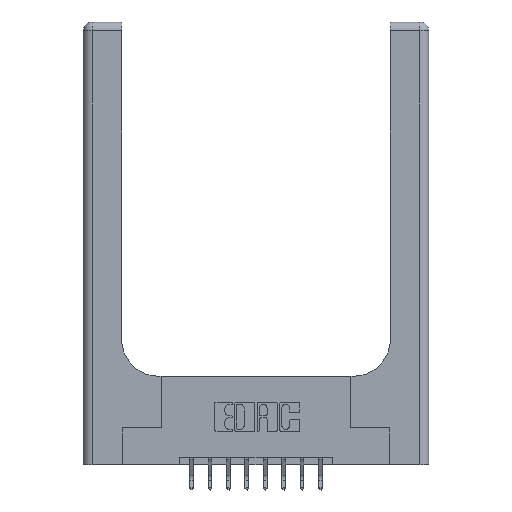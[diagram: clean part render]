
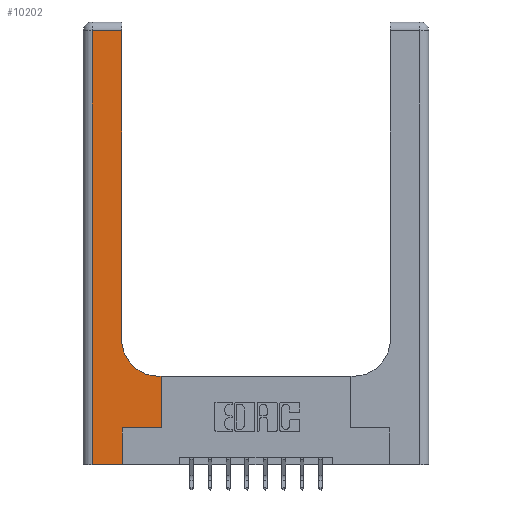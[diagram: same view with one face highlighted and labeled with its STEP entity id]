
A CAD part, top view. The second image highlights one B-rep face of the part: STEP entity #10202.
In plain terms, the highlighted planar face has unit normal (0, 0, 1).
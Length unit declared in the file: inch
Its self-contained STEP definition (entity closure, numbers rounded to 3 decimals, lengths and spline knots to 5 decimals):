
#303 = LINE ( 'NONE', #11230, #5489 ) ;
#729 = VECTOR ( 'NONE', #3623, 39.37008 ) ;
#952 = EDGE_CURVE ( 'NONE', #15078, #9808, #13751, .T. ) ;
#1310 = ORIENTED_EDGE ( 'NONE', *, *, #13194, .T. ) ;
#1444 = DIRECTION ( 'NONE',  ( 0., 1., 0. ) ) ;
#1522 = CARTESIAN_POINT ( 'NONE',  ( 0., 0., 0.37 ) ) ;
#1782 = CARTESIAN_POINT ( 'NONE',  ( 0.265, 0., 0.37 ) ) ;
#1829 = EDGE_CURVE ( 'NONE', #14123, #10329, #3282, .T. ) ;
#2497 = ORIENTED_EDGE ( 'NONE', *, *, #7614, .T. ) ;
#2545 = CARTESIAN_POINT ( 'NONE',  ( 0.265, 0.25, 0.37 ) ) ;
#2578 = EDGE_LOOP ( 'NONE', ( #7076, #1310, #2497, #11258, #5785, #10426, #13328, #14172, #7221 ) ) ;
#2720 = DIRECTION ( 'NONE',  ( 0., 1., 0. ) ) ;
#3282 = LINE ( 'NONE', #4971, #3464 ) ;
#3456 = CARTESIAN_POINT ( 'NONE',  ( 0.51, 0.6, 0.37 ) ) ;
#3464 = VECTOR ( 'NONE', #1444, 39.37008 ) ;
#3581 = VERTEX_POINT ( 'NONE', #14454 ) ;
#3623 = DIRECTION ( 'NONE',  ( 1., 0., 0. ) ) ;
#3848 = CIRCLE ( 'NONE', #10645, 0.25 ) ;
#4052 = CARTESIAN_POINT ( 'NONE',  ( 0.26, 0.6, 0.37 ) ) ;
#4129 = DIRECTION ( 'NONE',  ( 0., 1., 0. ) ) ;
#4152 = DIRECTION ( 'NONE',  ( -1., 0., 0. ) ) ;
#4184 = CARTESIAN_POINT ( 'NONE',  ( 0., 3., 0.37 ) ) ;
#4971 = CARTESIAN_POINT ( 'NONE',  ( 0.26, 3., 0.37 ) ) ;
#5489 = VECTOR ( 'NONE', #4129, 39.37008 ) ;
#5581 = CARTESIAN_POINT ( 'NONE',  ( 0.26, 2.94, 0.37 ) ) ;
#5785 = ORIENTED_EDGE ( 'NONE', *, *, #6440, .T. ) ;
#6237 = CARTESIAN_POINT ( 'NONE',  ( 0.528, 0.25, 0.37 ) ) ;
#6440 = EDGE_CURVE ( 'NONE', #6472, #15078, #303, .T. ) ;
#6472 = VERTEX_POINT ( 'NONE', #1782 ) ;
#6755 = AXIS2_PLACEMENT_3D ( 'NONE', #4184, #12388, #8921 ) ;
#6805 = CARTESIAN_POINT ( 'NONE',  ( 0.528, 0.6, 0.37 ) ) ;
#7043 = DIRECTION ( 'NONE',  ( 1., 0., 0. ) ) ;
#7076 = ORIENTED_EDGE ( 'NONE', *, *, #1829, .T. ) ;
#7221 = ORIENTED_EDGE ( 'NONE', *, *, #10772, .T. ) ;
#7222 = VECTOR ( 'NONE', #4152, 39.37008 ) ;
#7394 = FACE_OUTER_BOUND ( 'NONE', #2578, .T. ) ;
#7455 = DIRECTION ( 'NONE',  ( -1., 0., 0. ) ) ;
#7469 = DIRECTION ( 'NONE',  ( 0., -1., 0. ) ) ;
#7614 = EDGE_CURVE ( 'NONE', #3581, #13127, #10199, .T. ) ;
#7657 = DIRECTION ( 'NONE',  ( 1., 0., 0. ) ) ;
#8317 = LINE ( 'NONE', #4052, #7222 ) ;
#8325 = CARTESIAN_POINT ( 'NONE',  ( 0.528, 0.25, 0.37 ) ) ;
#8884 = CARTESIAN_POINT ( 'NONE',  ( 0.26, 0.85, 0.37 ) ) ;
#8921 = DIRECTION ( 'NONE',  ( -1., 0., 0. ) ) ;
#9393 = EDGE_CURVE ( 'NONE', #11562, #14294, #8317, .T. ) ;
#9660 = CARTESIAN_POINT ( 'NONE',  ( 0.06, 3., 0.37 ) ) ;
#9759 = CARTESIAN_POINT ( 'NONE',  ( 0., 2.94, 0.37 ) ) ;
#9808 = VERTEX_POINT ( 'NONE', #8325 ) ;
#10199 = LINE ( 'NONE', #9660, #11870 ) ;
#10202 = ADVANCED_FACE ( 'NONE', ( #7394 ), #11188, .F. ) ;
#10329 = VERTEX_POINT ( 'NONE', #5581 ) ;
#10426 = ORIENTED_EDGE ( 'NONE', *, *, #952, .T. ) ;
#10645 = AXIS2_PLACEMENT_3D ( 'NONE', #12807, #12859, #7043 ) ;
#10772 = EDGE_CURVE ( 'NONE', #14294, #14123, #3848, .T. ) ;
#11188 = PLANE ( 'NONE',  #6755 ) ;
#11230 = CARTESIAN_POINT ( 'NONE',  ( 0.265, 0., 0.37 ) ) ;
#11258 = ORIENTED_EDGE ( 'NONE', *, *, #14582, .T. ) ;
#11562 = VERTEX_POINT ( 'NONE', #6805 ) ;
#11677 = CARTESIAN_POINT ( 'NONE',  ( 0.265, 0.25, 0.37 ) ) ;
#11870 = VECTOR ( 'NONE', #7469, 39.37008 ) ;
#12375 = VECTOR ( 'NONE', #7657, 39.37008 ) ;
#12388 = DIRECTION ( 'NONE',  ( 0., 0., -1. ) ) ;
#12807 = CARTESIAN_POINT ( 'NONE',  ( 0.51, 0.85, 0.37 ) ) ;
#12859 = DIRECTION ( 'NONE',  ( 0., 0., -1. ) ) ;
#13098 = LINE ( 'NONE', #6237, #13461 ) ;
#13127 = VERTEX_POINT ( 'NONE', #14638 ) ;
#13194 = EDGE_CURVE ( 'NONE', #10329, #3581, #13651, .T. ) ;
#13328 = ORIENTED_EDGE ( 'NONE', *, *, #13518, .T. ) ;
#13461 = VECTOR ( 'NONE', #2720, 39.37008 ) ;
#13518 = EDGE_CURVE ( 'NONE', #9808, #11562, #13098, .T. ) ;
#13651 = LINE ( 'NONE', #9759, #14223 ) ;
#13751 = LINE ( 'NONE', #11677, #729 ) ;
#14123 = VERTEX_POINT ( 'NONE', #8884 ) ;
#14172 = ORIENTED_EDGE ( 'NONE', *, *, #9393, .T. ) ;
#14223 = VECTOR ( 'NONE', #7455, 39.37008 ) ;
#14294 = VERTEX_POINT ( 'NONE', #3456 ) ;
#14387 = LINE ( 'NONE', #1522, #12375 ) ;
#14454 = CARTESIAN_POINT ( 'NONE',  ( 0.06, 2.94, 0.37 ) ) ;
#14582 = EDGE_CURVE ( 'NONE', #13127, #6472, #14387, .T. ) ;
#14638 = CARTESIAN_POINT ( 'NONE',  ( 0.06, 0., 0.37 ) ) ;
#15078 = VERTEX_POINT ( 'NONE', #2545 ) ;
